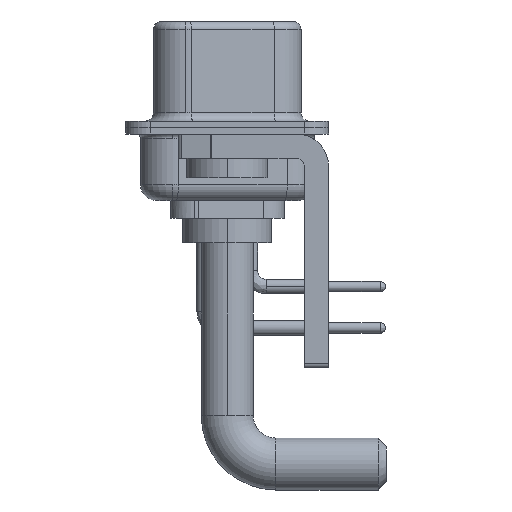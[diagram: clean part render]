
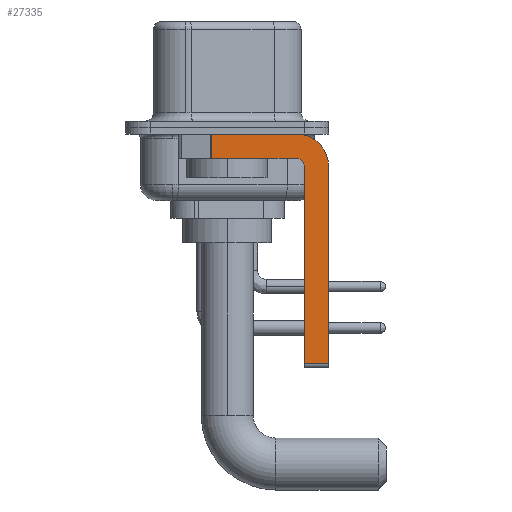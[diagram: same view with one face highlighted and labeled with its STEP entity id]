
A CAD part, left-side view. The second image highlights one B-rep face of the part: STEP entity #27335.
In plain terms, the highlighted planar face has unit normal (-1, 0, 0).
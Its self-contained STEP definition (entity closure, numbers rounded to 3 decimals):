
#206 = CIRCLE ( 'NONE', #12710, 0.5 ) ;
#1185 = EDGE_CURVE ( 'NONE', #13061, #27675, #18073, .T. ) ;
#1255 = ORIENTED_EDGE ( 'NONE', *, *, #1185, .F. ) ;
#2576 = LINE ( 'NONE', #19651, #26574 ) ;
#2780 = DIRECTION ( 'NONE',  ( -1., 0., 0. ) ) ;
#3030 = DIRECTION ( 'NONE',  ( 0., 0., -1. ) ) ;
#3585 = AXIS2_PLACEMENT_3D ( 'NONE', #13656, #4697, #3030 ) ;
#3752 = CARTESIAN_POINT ( 'NONE',  ( -2.9, -4.75, -14.55 ) ) ;
#4110 = CARTESIAN_POINT ( 'NONE',  ( -2.9, -6.25, -14.55 ) ) ;
#4154 = ORIENTED_EDGE ( 'NONE', *, *, #24729, .T. ) ;
#4697 = DIRECTION ( 'NONE',  ( 1., 0., 0. ) ) ;
#5772 = CARTESIAN_POINT ( 'NONE',  ( -2.9, -4.25, -1.9 ) ) ;
#8862 = VERTEX_POINT ( 'NONE', #10328 ) ;
#9291 = ORIENTED_EDGE ( 'NONE', *, *, #20522, .F. ) ;
#9431 = LINE ( 'NONE', #18394, #19935 ) ;
#9507 = ORIENTED_EDGE ( 'NONE', *, *, #10938, .F. ) ;
#9650 = EDGE_CURVE ( 'NONE', #23732, #20776, #9431, .T. ) ;
#9821 = ORIENTED_EDGE ( 'NONE', *, *, #17398, .F. ) ;
#10328 = CARTESIAN_POINT ( 'NONE',  ( -2.9, 0.978, -1.9 ) ) ;
#10637 = EDGE_CURVE ( 'NONE', #24337, #18692, #18729, .T. ) ;
#10835 = DIRECTION ( 'NONE',  ( 0., -1., 0. ) ) ;
#10938 = EDGE_CURVE ( 'NONE', #14022, #8862, #18721, .T. ) ;
#11044 = ORIENTED_EDGE ( 'NONE', *, *, #10637, .F. ) ;
#11550 = CARTESIAN_POINT ( 'NONE',  ( -2.9, 0.978, -0.4 ) ) ;
#12710 = AXIS2_PLACEMENT_3D ( 'NONE', #23759, #2780, #19854 ) ;
#12787 = VECTOR ( 'NONE', #25184, 1000. ) ;
#13061 = VERTEX_POINT ( 'NONE', #19158 ) ;
#13166 = ORIENTED_EDGE ( 'NONE', *, *, #16606, .T. ) ;
#13656 = CARTESIAN_POINT ( 'NONE',  ( -2.9, -4.25, -2.4 ) ) ;
#14022 = VERTEX_POINT ( 'NONE', #5772 ) ;
#14120 = FACE_OUTER_BOUND ( 'NONE', #15820, .T. ) ;
#14243 = DIRECTION ( 'NONE',  ( 0., 1., 0. ) ) ;
#15340 = VECTOR ( 'NONE', #10835, 1000. ) ;
#15458 = DIRECTION ( 'NONE',  ( 0., 0., -1. ) ) ;
#15528 = VECTOR ( 'NONE', #14243, 1000. ) ;
#15820 = EDGE_LOOP ( 'NONE', ( #11044, #4154, #9507, #9291, #27214, #13166, #1255, #9821 ) ) ;
#16178 = CIRCLE ( 'NONE', #26948, 2. ) ;
#16234 = CARTESIAN_POINT ( 'NONE',  ( -2.9, -6.25, -2.4 ) ) ;
#16277 = CARTESIAN_POINT ( 'NONE',  ( -2.9, -4.25, -2.4 ) ) ;
#16547 = DIRECTION ( 'NONE',  ( 1., 0., 0. ) ) ;
#16606 = EDGE_CURVE ( 'NONE', #23732, #27675, #24877, .T. ) ;
#16628 = CARTESIAN_POINT ( 'NONE',  ( -2.9, 3., -0.4 ) ) ;
#17398 = EDGE_CURVE ( 'NONE', #18692, #13061, #16178, .T. ) ;
#18073 = LINE ( 'NONE', #16234, #22143 ) ;
#18394 = CARTESIAN_POINT ( 'NONE',  ( -2.9, -4.75, -14.8 ) ) ;
#18692 = VERTEX_POINT ( 'NONE', #22396 ) ;
#18721 = LINE ( 'NONE', #21091, #15528 ) ;
#18729 = LINE ( 'NONE', #16628, #12787 ) ;
#19158 = CARTESIAN_POINT ( 'NONE',  ( -2.9, -6.25, -2.4 ) ) ;
#19651 = CARTESIAN_POINT ( 'NONE',  ( -2.9, 0.978, -1.9 ) ) ;
#19854 = DIRECTION ( 'NONE',  ( 0., 0., 1. ) ) ;
#19935 = VECTOR ( 'NONE', #22049, 1000. ) ;
#20522 = EDGE_CURVE ( 'NONE', #20776, #14022, #206, .T. ) ;
#20776 = VERTEX_POINT ( 'NONE', #21308 ) ;
#21019 = DIRECTION ( 'NONE',  ( 0., 0., -1. ) ) ;
#21091 = CARTESIAN_POINT ( 'NONE',  ( -2.9, -4.25, -1.9 ) ) ;
#21308 = CARTESIAN_POINT ( 'NONE',  ( -2.9, -4.75, -2.4 ) ) ;
#21902 = PLANE ( 'NONE',  #3585 ) ;
#22049 = DIRECTION ( 'NONE',  ( 0., 0., 1. ) ) ;
#22128 = DIRECTION ( 'NONE',  ( 0., 0., -1. ) ) ;
#22143 = VECTOR ( 'NONE', #22128, 1000. ) ;
#22396 = CARTESIAN_POINT ( 'NONE',  ( -2.9, -4.25, -0.4 ) ) ;
#23732 = VERTEX_POINT ( 'NONE', #3752 ) ;
#23759 = CARTESIAN_POINT ( 'NONE',  ( -2.9, -4.25, -2.4 ) ) ;
#24337 = VERTEX_POINT ( 'NONE', #11550 ) ;
#24729 = EDGE_CURVE ( 'NONE', #24337, #8862, #2576, .T. ) ;
#24877 = LINE ( 'NONE', #25294, #15340 ) ;
#25184 = DIRECTION ( 'NONE',  ( 0., -1., 0. ) ) ;
#25294 = CARTESIAN_POINT ( 'NONE',  ( -2.9, -4.25, -14.55 ) ) ;
#26574 = VECTOR ( 'NONE', #15458, 1000. ) ;
#26948 = AXIS2_PLACEMENT_3D ( 'NONE', #16277, #16547, #21019 ) ;
#27214 = ORIENTED_EDGE ( 'NONE', *, *, #9650, .F. ) ;
#27335 = ADVANCED_FACE ( 'NONE', ( #14120 ), #21902, .F. ) ;
#27675 = VERTEX_POINT ( 'NONE', #4110 ) ;
